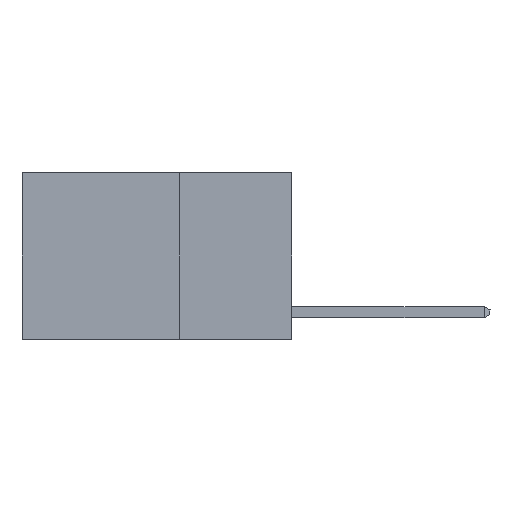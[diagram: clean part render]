
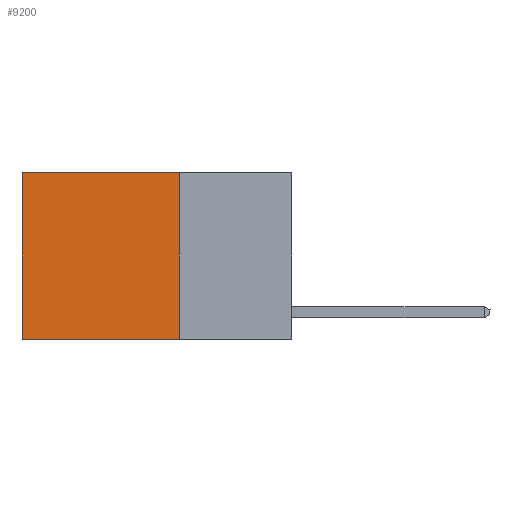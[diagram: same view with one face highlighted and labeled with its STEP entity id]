
A CAD part, left-side view. The second image highlights one B-rep face of the part: STEP entity #9200.
In plain terms, the highlighted planar face has unit normal (-1, 0, 0).
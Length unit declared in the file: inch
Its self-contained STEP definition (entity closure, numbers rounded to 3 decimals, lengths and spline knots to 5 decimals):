
#4 = DIRECTION ( 'NONE',  ( 0., 0., -1. ) ) ;
#464 = DIRECTION ( 'NONE',  ( 0., 1., 0. ) ) ;
#1108 = EDGE_CURVE ( 'NONE', #4874, #17464, #5321, .T. ) ;
#1682 = ORIENTED_EDGE ( 'NONE', *, *, #13209, .F. ) ;
#1771 = VERTEX_POINT ( 'NONE', #4503 ) ;
#1785 = EDGE_CURVE ( 'NONE', #6425, #1771, #16348, .T. ) ;
#2207 = EDGE_CURVE ( 'NONE', #17464, #1771, #12163, .T. ) ;
#2447 = EDGE_LOOP ( 'NONE', ( #3049, #3183, #1682, #13094 ) ) ;
#2543 = CARTESIAN_POINT ( 'NONE',  ( 0.2625, 0.25, 0. ) ) ;
#3049 = ORIENTED_EDGE ( 'NONE', *, *, #2207, .T. ) ;
#3183 = ORIENTED_EDGE ( 'NONE', *, *, #1785, .F. ) ;
#3908 = VECTOR ( 'NONE', #4, 39.37008 ) ;
#4128 = PLANE ( 'NONE',  #6637 ) ;
#4503 = CARTESIAN_POINT ( 'NONE',  ( 0.2625, 0.6, -0.37 ) ) ;
#4789 = DIRECTION ( 'NONE',  ( 0., 1., 0. ) ) ;
#4874 = VERTEX_POINT ( 'NONE', #16956 ) ;
#5321 = LINE ( 'NONE', #9503, #18850 ) ;
#5435 = CARTESIAN_POINT ( 'NONE',  ( 0.2625, 0.25, -0.37 ) ) ;
#6324 = LINE ( 'NONE', #10781, #3908 ) ;
#6425 = VERTEX_POINT ( 'NONE', #5435 ) ;
#6637 = AXIS2_PLACEMENT_3D ( 'NONE', #2543, #14426, #7131 ) ;
#6690 = VECTOR ( 'NONE', #12259, 39.37008 ) ;
#7131 = DIRECTION ( 'NONE',  ( 0., 0., -1. ) ) ;
#7804 = CARTESIAN_POINT ( 'NONE',  ( 0.2625, 0.25, -0.37 ) ) ;
#8746 = VECTOR ( 'NONE', #4789, 39.37008 ) ;
#9200 = ADVANCED_FACE ( 'NONE', ( #17220 ), #4128, .F. ) ;
#9503 = CARTESIAN_POINT ( 'NONE',  ( 0.2625, 0.25, 0. ) ) ;
#10781 = CARTESIAN_POINT ( 'NONE',  ( 0.2625, 0.25, 0. ) ) ;
#12163 = LINE ( 'NONE', #16735, #6690 ) ;
#12259 = DIRECTION ( 'NONE',  ( 0., 0., -1. ) ) ;
#13094 = ORIENTED_EDGE ( 'NONE', *, *, #1108, .T. ) ;
#13209 = EDGE_CURVE ( 'NONE', #4874, #6425, #6324, .T. ) ;
#14426 = DIRECTION ( 'NONE',  ( 1., 0., 0. ) ) ;
#15460 = CARTESIAN_POINT ( 'NONE',  ( 0.2625, 0.6, 0. ) ) ;
#16348 = LINE ( 'NONE', #7804, #8746 ) ;
#16735 = CARTESIAN_POINT ( 'NONE',  ( 0.2625, 0.6, 0. ) ) ;
#16956 = CARTESIAN_POINT ( 'NONE',  ( 0.2625, 0.25, 0. ) ) ;
#17220 = FACE_OUTER_BOUND ( 'NONE', #2447, .T. ) ;
#17464 = VERTEX_POINT ( 'NONE', #15460 ) ;
#18850 = VECTOR ( 'NONE', #464, 39.37008 ) ;
